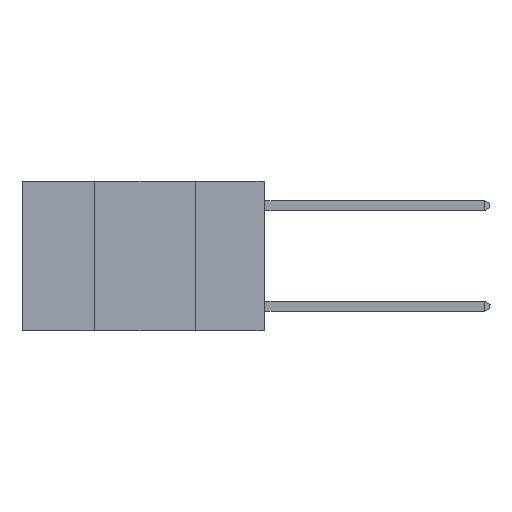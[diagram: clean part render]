
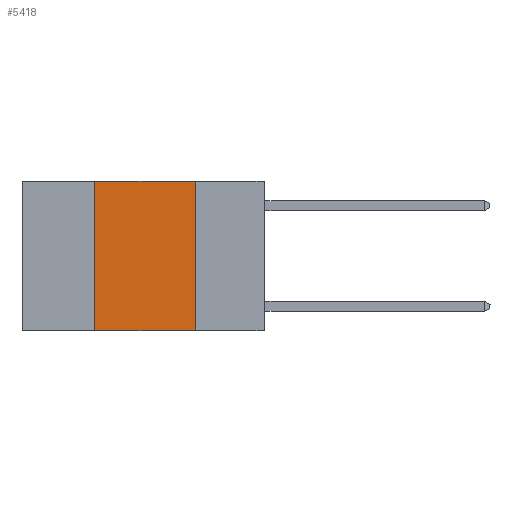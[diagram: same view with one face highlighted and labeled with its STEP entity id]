
A CAD part, left-side view. The second image highlights one B-rep face of the part: STEP entity #5418.
In plain terms, the highlighted planar face has unit normal (-1, 0, 0).
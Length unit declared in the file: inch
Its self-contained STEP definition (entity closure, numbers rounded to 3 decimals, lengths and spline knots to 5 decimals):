
#323 = ORIENTED_EDGE ( 'NONE', *, *, #6252, .F. ) ;
#505 = VERTEX_POINT ( 'NONE', #7914 ) ;
#514 = CARTESIAN_POINT ( 'NONE',  ( 0., 0.17, 0. ) ) ;
#634 = ORIENTED_EDGE ( 'NONE', *, *, #983, .F. ) ;
#983 = EDGE_CURVE ( 'NONE', #1158, #5038, #8166, .T. ) ;
#1158 = VERTEX_POINT ( 'NONE', #7397 ) ;
#1282 = LINE ( 'NONE', #9843, #10529 ) ;
#1865 = DIRECTION ( 'NONE',  ( 0., 0., 1. ) ) ;
#2365 = VECTOR ( 'NONE', #10436, 39.37008 ) ;
#3048 = VECTOR ( 'NONE', #1865, 39.37008 ) ;
#3383 = PLANE ( 'NONE',  #4113 ) ;
#4113 = AXIS2_PLACEMENT_3D ( 'NONE', #7055, #9713, #4337 ) ;
#4337 = DIRECTION ( 'NONE',  ( 0., 0., -1. ) ) ;
#5038 = VERTEX_POINT ( 'NONE', #8159 ) ;
#5074 = FACE_OUTER_BOUND ( 'NONE', #10844, .T. ) ;
#5339 = VECTOR ( 'NONE', #7101, 39.37008 ) ;
#5418 = ADVANCED_FACE ( 'NONE', ( #5074 ), #3383, .F. ) ;
#5612 = ORIENTED_EDGE ( 'NONE', *, *, #11569, .T. ) ;
#6252 = EDGE_CURVE ( 'NONE', #5038, #9784, #1282, .T. ) ;
#6340 = DIRECTION ( 'NONE',  ( 0., -1., 0. ) ) ;
#6961 = EDGE_CURVE ( 'NONE', #9784, #505, #7384, .T. ) ;
#7055 = CARTESIAN_POINT ( 'NONE',  ( 0., 0.6, 0. ) ) ;
#7101 = DIRECTION ( 'NONE',  ( 0., 0., -1. ) ) ;
#7384 = LINE ( 'NONE', #9721, #5339 ) ;
#7397 = CARTESIAN_POINT ( 'NONE',  ( 0., 0.42, -0.37 ) ) ;
#7914 = CARTESIAN_POINT ( 'NONE',  ( 0., 0.17, -0.37 ) ) ;
#8159 = CARTESIAN_POINT ( 'NONE',  ( 0., 0.42, 0. ) ) ;
#8166 = LINE ( 'NONE', #10771, #3048 ) ;
#9569 = LINE ( 'NONE', #9607, #2365 ) ;
#9607 = CARTESIAN_POINT ( 'NONE',  ( 0., 0.6, -0.37 ) ) ;
#9713 = DIRECTION ( 'NONE',  ( 1., 0., 0. ) ) ;
#9721 = CARTESIAN_POINT ( 'NONE',  ( 0., 0.17, 0. ) ) ;
#9740 = ORIENTED_EDGE ( 'NONE', *, *, #6961, .F. ) ;
#9784 = VERTEX_POINT ( 'NONE', #514 ) ;
#9843 = CARTESIAN_POINT ( 'NONE',  ( 0., 0.6, 0. ) ) ;
#10436 = DIRECTION ( 'NONE',  ( 0., -1., 0. ) ) ;
#10529 = VECTOR ( 'NONE', #6340, 39.37008 ) ;
#10771 = CARTESIAN_POINT ( 'NONE',  ( 0., 0.42, 0. ) ) ;
#10844 = EDGE_LOOP ( 'NONE', ( #9740, #323, #634, #5612 ) ) ;
#11569 = EDGE_CURVE ( 'NONE', #1158, #505, #9569, .T. ) ;
